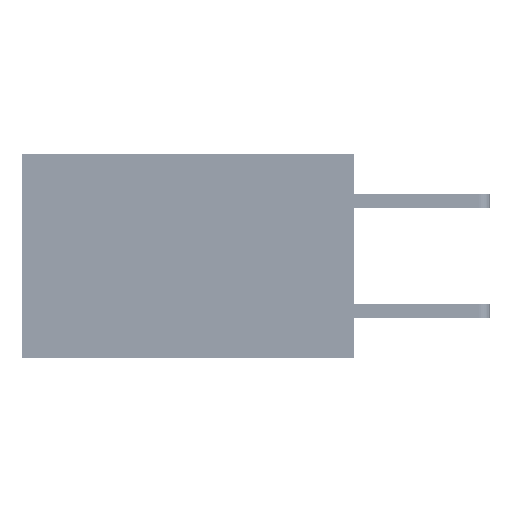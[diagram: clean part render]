
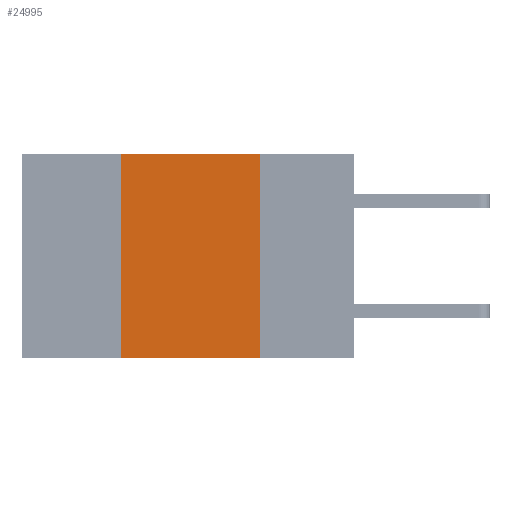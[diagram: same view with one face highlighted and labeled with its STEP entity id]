
A CAD part, left-side view. The second image highlights one B-rep face of the part: STEP entity #24995.
In plain terms, the highlighted planar face has unit normal (-1, 0, 0).
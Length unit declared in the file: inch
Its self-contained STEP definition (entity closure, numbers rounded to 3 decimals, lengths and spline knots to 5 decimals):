
#1246 = DIRECTION ( 'NONE',  ( 0., -1., 0. ) ) ;
#1836 = VECTOR ( 'NONE', #8728, 39.37008 ) ;
#2492 = ORIENTED_EDGE ( 'NONE', *, *, #33055, .F. ) ;
#3051 = CARTESIAN_POINT ( 'NONE',  ( 0., 0.42, -0.37 ) ) ;
#3222 = PLANE ( 'NONE',  #35409 ) ;
#5393 = VECTOR ( 'NONE', #1246, 39.37008 ) ;
#6406 = VERTEX_POINT ( 'NONE', #3051 ) ;
#7166 = FACE_OUTER_BOUND ( 'NONE', #32025, .T. ) ;
#7184 = CARTESIAN_POINT ( 'NONE',  ( 0., 0.6, 0. ) ) ;
#8728 = DIRECTION ( 'NONE',  ( 0., 0., -1. ) ) ;
#9183 = DIRECTION ( 'NONE',  ( 0., -1., 0. ) ) ;
#9228 = VERTEX_POINT ( 'NONE', #24603 ) ;
#9502 = EDGE_CURVE ( 'NONE', #6406, #14537, #16674, .T. ) ;
#12246 = LINE ( 'NONE', #15347, #1836 ) ;
#13227 = LINE ( 'NONE', #27245, #16532 ) ;
#13763 = DIRECTION ( 'NONE',  ( 1., 0., 0. ) ) ;
#14537 = VERTEX_POINT ( 'NONE', #15162 ) ;
#15162 = CARTESIAN_POINT ( 'NONE',  ( 0., 0.17, -0.37 ) ) ;
#15347 = CARTESIAN_POINT ( 'NONE',  ( 0., 0.17, 0. ) ) ;
#16532 = VECTOR ( 'NONE', #40675, 39.37008 ) ;
#16646 = CARTESIAN_POINT ( 'NONE',  ( 0., 0.6, 0. ) ) ;
#16674 = LINE ( 'NONE', #39550, #37449 ) ;
#21232 = LINE ( 'NONE', #7184, #5393 ) ;
#24603 = CARTESIAN_POINT ( 'NONE',  ( 0., 0.42, 0. ) ) ;
#24995 = ADVANCED_FACE ( 'NONE', ( #7166 ), #3222, .F. ) ;
#27189 = DIRECTION ( 'NONE',  ( 0., 0., -1. ) ) ;
#27245 = CARTESIAN_POINT ( 'NONE',  ( 0., 0.42, 0. ) ) ;
#32025 = EDGE_LOOP ( 'NONE', ( #32720, #42842, #2492, #40031 ) ) ;
#32720 = ORIENTED_EDGE ( 'NONE', *, *, #42360, .F. ) ;
#33055 = EDGE_CURVE ( 'NONE', #6406, #9228, #13227, .T. ) ;
#35409 = AXIS2_PLACEMENT_3D ( 'NONE', #16646, #13763, #27189 ) ;
#37449 = VECTOR ( 'NONE', #9183, 39.37008 ) ;
#39550 = CARTESIAN_POINT ( 'NONE',  ( 0., 0.6, -0.37 ) ) ;
#40031 = ORIENTED_EDGE ( 'NONE', *, *, #9502, .T. ) ;
#40675 = DIRECTION ( 'NONE',  ( 0., 0., 1. ) ) ;
#40825 = CARTESIAN_POINT ( 'NONE',  ( 0., 0.17, 0. ) ) ;
#41222 = VERTEX_POINT ( 'NONE', #40825 ) ;
#42360 = EDGE_CURVE ( 'NONE', #41222, #14537, #12246, .T. ) ;
#42842 = ORIENTED_EDGE ( 'NONE', *, *, #42975, .F. ) ;
#42975 = EDGE_CURVE ( 'NONE', #9228, #41222, #21232, .T. ) ;
